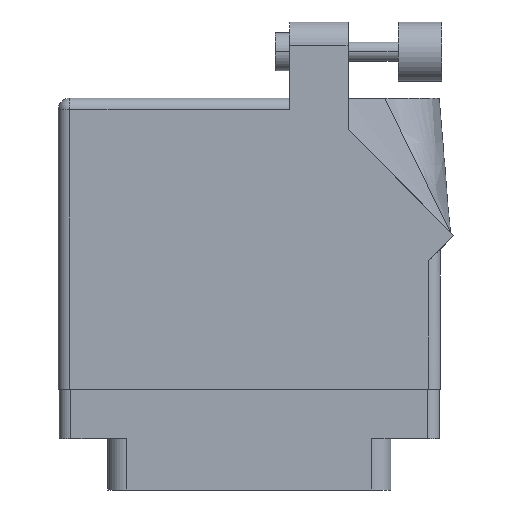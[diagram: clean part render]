
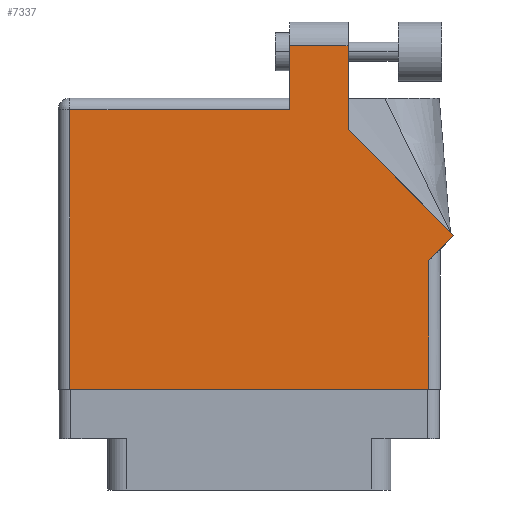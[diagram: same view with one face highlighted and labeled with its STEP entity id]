
A CAD part, front view. The second image highlights one B-rep face of the part: STEP entity #7337.
In plain terms, the highlighted face is planar.
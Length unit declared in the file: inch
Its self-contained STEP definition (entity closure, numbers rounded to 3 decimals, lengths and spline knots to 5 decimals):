
#627 = LINE ( 'NONE', #1880, #23095 ) ;
#908 = VERTEX_POINT ( 'NONE', #35139 ) ;
#1018 = DIRECTION ( 'NONE',  ( 0.707, 0.707, 0. ) ) ;
#1880 = CARTESIAN_POINT ( 'NONE',  ( 1.948, 0.737, 0. ) ) ;
#2818 = VERTEX_POINT ( 'NONE', #14128 ) ;
#4279 = VECTOR ( 'NONE', #30715, 39.37008 ) ;
#4926 = EDGE_CURVE ( 'NONE', #27889, #2818, #24001, .T. ) ;
#5637 = VERTEX_POINT ( 'NONE', #27808 ) ;
#5672 = VERTEX_POINT ( 'NONE', #15299 ) ;
#7279 = EDGE_CURVE ( 'NONE', #5637, #11803, #31445, .T. ) ;
#7337 = ADVANCED_FACE ( 'NONE', ( #14439 ), #14849, .F. ) ;
#7441 = EDGE_CURVE ( 'NONE', #11803, #24150, #32361, .T. ) ;
#7785 = VECTOR ( 'NONE', #37864, 39.37008 ) ;
#9421 = CARTESIAN_POINT ( 'NONE',  ( 1.948, 0., 0. ) ) ;
#9925 = CARTESIAN_POINT ( 'NONE',  ( 0., 1.468, 0. ) ) ;
#10298 = ORIENTED_EDGE ( 'NONE', *, *, #21677, .T. ) ;
#11178 = VECTOR ( 'NONE', #26028, 39.37008 ) ;
#11803 = VERTEX_POINT ( 'NONE', #27956 ) ;
#12530 = VERTEX_POINT ( 'NONE', #30936 ) ;
#13643 = CARTESIAN_POINT ( 'NONE',  ( 1.217, 1.53, 0. ) ) ;
#14073 = ORIENTED_EDGE ( 'NONE', *, *, #7279, .T. ) ;
#14128 = CARTESIAN_POINT ( 'NONE',  ( 1.524, 1.36442, 0. ) ) ;
#14439 = FACE_OUTER_BOUND ( 'NONE', #16685, .T. ) ;
#14849 = PLANE ( 'NONE',  #22951 ) ;
#14967 = VECTOR ( 'NONE', #19713, 39.37008 ) ;
#15002 = EDGE_CURVE ( 'NONE', #2818, #35473, #24579, .T. ) ;
#15299 = CARTESIAN_POINT ( 'NONE',  ( 1.217, 1.805, 0. ) ) ;
#15804 = ORIENTED_EDGE ( 'NONE', *, *, #38753, .T. ) ;
#15879 = LINE ( 'NONE', #17850, #22421 ) ;
#16611 = VECTOR ( 'NONE', #23329, 39.37008 ) ;
#16685 = EDGE_LOOP ( 'NONE', ( #17731, #10298, #18302, #15804, #14073, #27734, #19340, #20175, #28468 ) ) ;
#16732 = CARTESIAN_POINT ( 'NONE',  ( 1.217, 1.805, 0. ) ) ;
#17708 = CARTESIAN_POINT ( 'NONE',  ( 0., 1.53, 0. ) ) ;
#17731 = ORIENTED_EDGE ( 'NONE', *, *, #15002, .T. ) ;
#17850 = CARTESIAN_POINT ( 'NONE',  ( 2.01, 0.737, 0. ) ) ;
#18012 = CARTESIAN_POINT ( 'NONE',  ( 2.08071, 0.80771, 0. ) ) ;
#18302 = ORIENTED_EDGE ( 'NONE', *, *, #19534, .T. ) ;
#19340 = ORIENTED_EDGE ( 'NONE', *, *, #37759, .T. ) ;
#19534 = EDGE_CURVE ( 'NONE', #5672, #12530, #28982, .T. ) ;
#19713 = DIRECTION ( 'NONE',  ( -1., 0., 0. ) ) ;
#20175 = ORIENTED_EDGE ( 'NONE', *, *, #34569, .T. ) ;
#20427 = CARTESIAN_POINT ( 'NONE',  ( 1.524, 1.36442, 0. ) ) ;
#20454 = DIRECTION ( 'NONE',  ( 1., 0., 0. ) ) ;
#21677 = EDGE_CURVE ( 'NONE', #35473, #5672, #28642, .T. ) ;
#22421 = VECTOR ( 'NONE', #1018, 39.37008 ) ;
#22951 = AXIS2_PLACEMENT_3D ( 'NONE', #17708, #32627, #26687 ) ;
#23095 = VECTOR ( 'NONE', #31453, 39.37008 ) ;
#23329 = DIRECTION ( 'NONE',  ( 0., 1., 0. ) ) ;
#24001 = LINE ( 'NONE', #18012, #24957 ) ;
#24150 = VERTEX_POINT ( 'NONE', #9421 ) ;
#24579 = LINE ( 'NONE', #20427, #16611 ) ;
#24957 = VECTOR ( 'NONE', #33306, 39.37008 ) ;
#26028 = DIRECTION ( 'NONE',  ( 0., -1., 0. ) ) ;
#26294 = CARTESIAN_POINT ( 'NONE',  ( 0.062, 0., 0. ) ) ;
#26687 = DIRECTION ( 'NONE',  ( -1., 0., 0. ) ) ;
#27734 = ORIENTED_EDGE ( 'NONE', *, *, #7441, .T. ) ;
#27808 = CARTESIAN_POINT ( 'NONE',  ( 0.062, 1.468, 0. ) ) ;
#27889 = VERTEX_POINT ( 'NONE', #34460 ) ;
#27956 = CARTESIAN_POINT ( 'NONE',  ( 0.062, 0., 0. ) ) ;
#28468 = ORIENTED_EDGE ( 'NONE', *, *, #4926, .T. ) ;
#28642 = LINE ( 'NONE', #16732, #14967 ) ;
#28735 = CARTESIAN_POINT ( 'NONE',  ( 1.524, 1.805, 0. ) ) ;
#28982 = LINE ( 'NONE', #13643, #7785 ) ;
#30715 = DIRECTION ( 'NONE',  ( -1., 0., 0. ) ) ;
#30936 = CARTESIAN_POINT ( 'NONE',  ( 1.217, 1.468, 0. ) ) ;
#31445 = LINE ( 'NONE', #26294, #11178 ) ;
#31453 = DIRECTION ( 'NONE',  ( 0., 1., 0. ) ) ;
#32361 = LINE ( 'NONE', #38948, #36157 ) ;
#32627 = DIRECTION ( 'NONE',  ( 0., 0., -1. ) ) ;
#33306 = DIRECTION ( 'NONE',  ( -0.707, 0.707, 0. ) ) ;
#34460 = CARTESIAN_POINT ( 'NONE',  ( 2.08071, 0.80771, 0. ) ) ;
#34569 = EDGE_CURVE ( 'NONE', #908, #27889, #15879, .T. ) ;
#35139 = CARTESIAN_POINT ( 'NONE',  ( 1.948, 0.675, 0. ) ) ;
#35473 = VERTEX_POINT ( 'NONE', #28735 ) ;
#36157 = VECTOR ( 'NONE', #20454, 39.37008 ) ;
#36326 = LINE ( 'NONE', #9925, #4279 ) ;
#37759 = EDGE_CURVE ( 'NONE', #24150, #908, #627, .T. ) ;
#37864 = DIRECTION ( 'NONE',  ( 0., -1., 0. ) ) ;
#38753 = EDGE_CURVE ( 'NONE', #12530, #5637, #36326, .T. ) ;
#38948 = CARTESIAN_POINT ( 'NONE',  ( 0., 0., 0. ) ) ;
